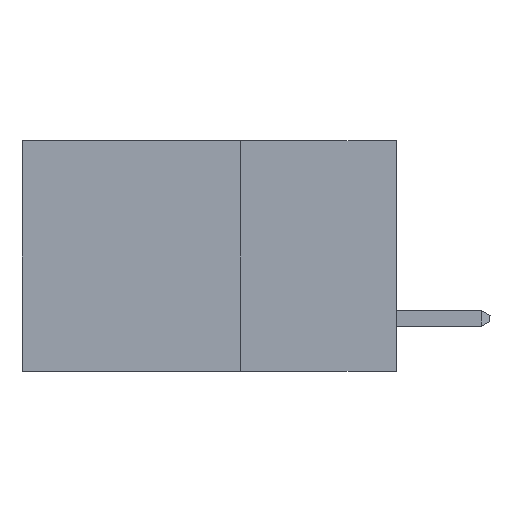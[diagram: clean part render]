
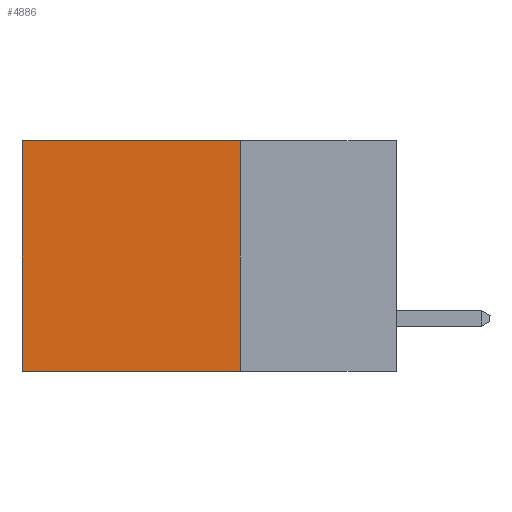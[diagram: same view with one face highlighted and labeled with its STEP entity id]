
A CAD part, left-side view. The second image highlights one B-rep face of the part: STEP entity #4886.
In plain terms, the highlighted planar face has unit normal (-1, 0, 0).
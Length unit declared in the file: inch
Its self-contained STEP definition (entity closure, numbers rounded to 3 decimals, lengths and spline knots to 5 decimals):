
#1703 = CARTESIAN_POINT ( 'NONE',  ( 0.2615, 0.6, -0.37 ) ) ;
#2119 = VERTEX_POINT ( 'NONE', #13037 ) ;
#2180 = LINE ( 'NONE', #3718, #2332 ) ;
#2273 = DIRECTION ( 'NONE',  ( 0., 0., -1. ) ) ;
#2332 = VECTOR ( 'NONE', #8830, 39.37008 ) ;
#2598 = CARTESIAN_POINT ( 'NONE',  ( 0.2615, 0.25, -0.37 ) ) ;
#3325 = EDGE_CURVE ( 'NONE', #10606, #11707, #2180, .T. ) ;
#3500 = CARTESIAN_POINT ( 'NONE',  ( 0.2615, 0.6, 0. ) ) ;
#3718 = CARTESIAN_POINT ( 'NONE',  ( 0.2615, 0.6, -0.37 ) ) ;
#3969 = CARTESIAN_POINT ( 'NONE',  ( 0.2615, 0.25, -0.37 ) ) ;
#4404 = CARTESIAN_POINT ( 'NONE',  ( 0.2615, 0.25, -0.37 ) ) ;
#4886 = ADVANCED_FACE ( 'NONE', ( #15090 ), #9688, .F. ) ;
#4891 = LINE ( 'NONE', #10167, #5853 ) ;
#4987 = VECTOR ( 'NONE', #13475, 39.37008 ) ;
#5197 = ORIENTED_EDGE ( 'NONE', *, *, #3325, .T. ) ;
#5595 = EDGE_CURVE ( 'NONE', #8309, #11707, #8242, .T. ) ;
#5853 = VECTOR ( 'NONE', #11724, 39.37008 ) ;
#6378 = EDGE_CURVE ( 'NONE', #2119, #10606, #4891, .T. ) ;
#7372 = VECTOR ( 'NONE', #2273, 39.37008 ) ;
#8242 = LINE ( 'NONE', #3969, #4987 ) ;
#8309 = VERTEX_POINT ( 'NONE', #13736 ) ;
#8830 = DIRECTION ( 'NONE',  ( 0., 0., -1. ) ) ;
#8844 = LINE ( 'NONE', #2598, #7372 ) ;
#9184 = ORIENTED_EDGE ( 'NONE', *, *, #16347, .F. ) ;
#9688 = PLANE ( 'NONE',  #12905 ) ;
#10167 = CARTESIAN_POINT ( 'NONE',  ( 0.2615, 0.25, 0. ) ) ;
#10606 = VERTEX_POINT ( 'NONE', #3500 ) ;
#11069 = DIRECTION ( 'NONE',  ( 1., 0., 0. ) ) ;
#11707 = VERTEX_POINT ( 'NONE', #1703 ) ;
#11724 = DIRECTION ( 'NONE',  ( 0., 1., 0. ) ) ;
#11910 = ORIENTED_EDGE ( 'NONE', *, *, #5595, .F. ) ;
#11993 = ORIENTED_EDGE ( 'NONE', *, *, #6378, .T. ) ;
#12905 = AXIS2_PLACEMENT_3D ( 'NONE', #4404, #11069, #13786 ) ;
#13037 = CARTESIAN_POINT ( 'NONE',  ( 0.2615, 0.25, 0. ) ) ;
#13475 = DIRECTION ( 'NONE',  ( 0., 1., 0. ) ) ;
#13736 = CARTESIAN_POINT ( 'NONE',  ( 0.2615, 0.25, -0.37 ) ) ;
#13786 = DIRECTION ( 'NONE',  ( 0., 0., -1. ) ) ;
#15090 = FACE_OUTER_BOUND ( 'NONE', #15150, .T. ) ;
#15150 = EDGE_LOOP ( 'NONE', ( #5197, #11910, #9184, #11993 ) ) ;
#16347 = EDGE_CURVE ( 'NONE', #2119, #8309, #8844, .T. ) ;
